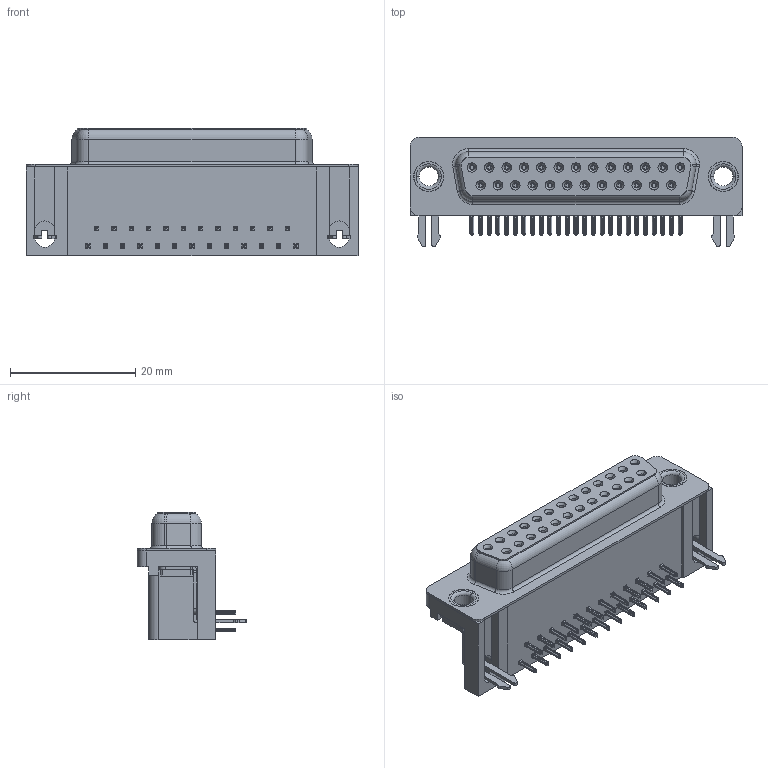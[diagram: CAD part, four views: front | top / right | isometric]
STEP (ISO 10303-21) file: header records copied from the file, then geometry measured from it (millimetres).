
FILE_DESCRIPTION (( 'STEP AP203' ), '1' );
FILE_NAME ('630-025-640-031.STEP', '2021-09-22T14:09:09', ( '' ), ( '' ), 'SwSTEP 2.0', 'SolidWorks 2020', '' );
FILE_SCHEMA (( 'CONFIG_CONTROL_DESIGN' ));
Length unit declared in the file: millimetre
Products named in the file (7): 630 Housing_25 Socket; 630 Shell_25 Socket; 630 Contact Bottom; 630 Thru Hole Rivet; 630 Contact Top; 630 2 Prong Board Lock; 630-025-640-031
Assembly tree (31 placements, depth 2):
  630-025-640-031
    630 Housing_25 Socket
    630 Shell_25 Socket
    630 Contact Bottom  x12
    630 Contact Top  x13
    630 2 Prong Board Lock  x2
    630 Thru Hole Rivet  x2
Bounding box: 53.04 x 17.48 x 20.4 mm (x, y, z)
Volume: 8580 mm3; surface area: 10087.8 mm2
Topology: 31 solids, 31 shells, 3850 faces, 10112 edges, 6344 vertices
Faces by surface type: plane 1754, cylinder 910, bspline 852, cone 300, torus 34
Entity records: 29268 total; most frequent: CARTESIAN_POINT 7934, ORIENTED_EDGE 4220, DIRECTION 3918, EDGE_CURVE 2110, LINE 1404, VECTOR 1404, VERTEX_POINT 1348, AXIS2_PLACEMENT_3D 1257
